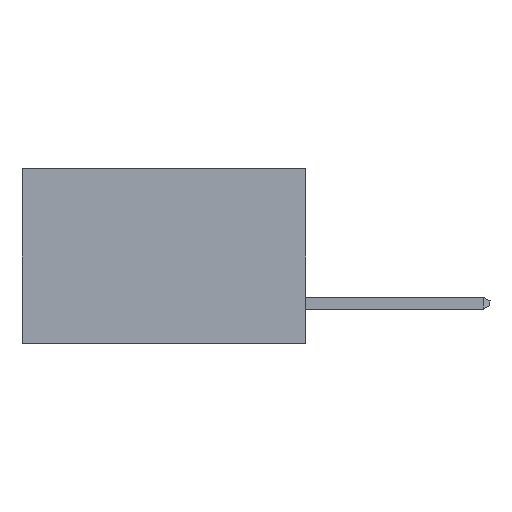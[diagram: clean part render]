
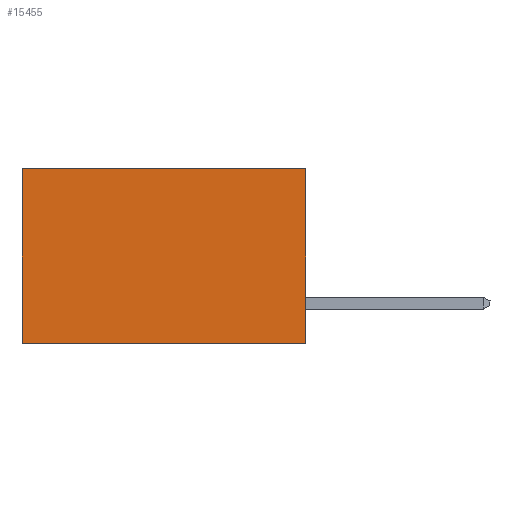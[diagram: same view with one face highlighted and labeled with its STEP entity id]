
A CAD part, left-side view. The second image highlights one B-rep face of the part: STEP entity #15455.
In plain terms, the highlighted planar face has unit normal (-1, 0, 0).
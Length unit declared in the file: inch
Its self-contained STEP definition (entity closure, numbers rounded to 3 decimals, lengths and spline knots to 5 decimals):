
#140 = DIRECTION ( 'NONE',  ( 0., 1., 0. ) ) ;
#1033 = DIRECTION ( 'NONE',  ( 0., 0., -1. ) ) ;
#1389 = CARTESIAN_POINT ( 'NONE',  ( 0.2615, 0., 0. ) ) ;
#1393 = DIRECTION ( 'NONE',  ( 0., 0., -1. ) ) ;
#1696 = CARTESIAN_POINT ( 'NONE',  ( 0.2615, 0., -0.37 ) ) ;
#2288 = ORIENTED_EDGE ( 'NONE', *, *, #5713, .F. ) ;
#2722 = EDGE_CURVE ( 'NONE', #4631, #4369, #6596, .T. ) ;
#4369 = VERTEX_POINT ( 'NONE', #7728 ) ;
#4477 = ORIENTED_EDGE ( 'NONE', *, *, #2722, .F. ) ;
#4526 = LINE ( 'NONE', #12607, #12057 ) ;
#4631 = VERTEX_POINT ( 'NONE', #1696 ) ;
#4976 = CARTESIAN_POINT ( 'NONE',  ( 0.2615, 0.6, 0. ) ) ;
#5115 = PLANE ( 'NONE',  #14930 ) ;
#5713 = EDGE_CURVE ( 'NONE', #5946, #4631, #4526, .T. ) ;
#5946 = VERTEX_POINT ( 'NONE', #1389 ) ;
#6359 = LINE ( 'NONE', #9158, #9666 ) ;
#6596 = LINE ( 'NONE', #12070, #7048 ) ;
#6608 = VECTOR ( 'NONE', #1393, 39.37008 ) ;
#6970 = ORIENTED_EDGE ( 'NONE', *, *, #16251, .T. ) ;
#7048 = VECTOR ( 'NONE', #140, 39.37008 ) ;
#7657 = FACE_OUTER_BOUND ( 'NONE', #12802, .T. ) ;
#7728 = CARTESIAN_POINT ( 'NONE',  ( 0.2615, 0.6, -0.37 ) ) ;
#8097 = LINE ( 'NONE', #11924, #6608 ) ;
#9158 = CARTESIAN_POINT ( 'NONE',  ( 0.2615, 0., 0. ) ) ;
#9666 = VECTOR ( 'NONE', #12791, 39.37008 ) ;
#9837 = VERTEX_POINT ( 'NONE', #4976 ) ;
#11242 = DIRECTION ( 'NONE',  ( 0., 0., -1. ) ) ;
#11924 = CARTESIAN_POINT ( 'NONE',  ( 0.2615, 0.6, -0.37 ) ) ;
#12057 = VECTOR ( 'NONE', #11242, 39.37008 ) ;
#12070 = CARTESIAN_POINT ( 'NONE',  ( 0.2615, 0., -0.37 ) ) ;
#12607 = CARTESIAN_POINT ( 'NONE',  ( 0.2615, 0., -0.37 ) ) ;
#12791 = DIRECTION ( 'NONE',  ( 0., 1., 0. ) ) ;
#12802 = EDGE_LOOP ( 'NONE', ( #16762, #4477, #2288, #6970 ) ) ;
#12958 = DIRECTION ( 'NONE',  ( 1., 0., 0. ) ) ;
#14930 = AXIS2_PLACEMENT_3D ( 'NONE', #16979, #12958, #1033 ) ;
#15455 = ADVANCED_FACE ( 'NONE', ( #7657 ), #5115, .F. ) ;
#16251 = EDGE_CURVE ( 'NONE', #5946, #9837, #6359, .T. ) ;
#16328 = EDGE_CURVE ( 'NONE', #9837, #4369, #8097, .T. ) ;
#16762 = ORIENTED_EDGE ( 'NONE', *, *, #16328, .T. ) ;
#16979 = CARTESIAN_POINT ( 'NONE',  ( 0.2615, 0., -0.37 ) ) ;
